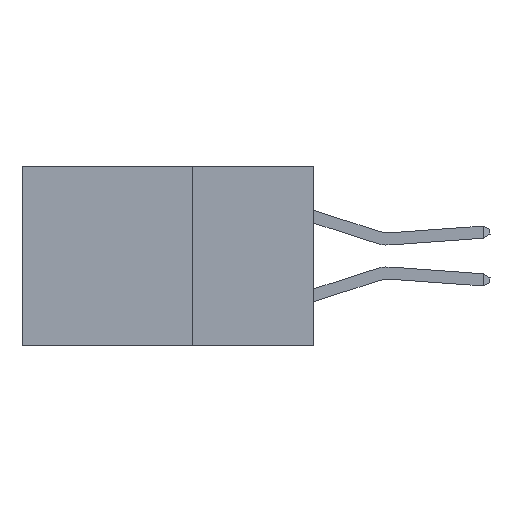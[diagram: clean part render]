
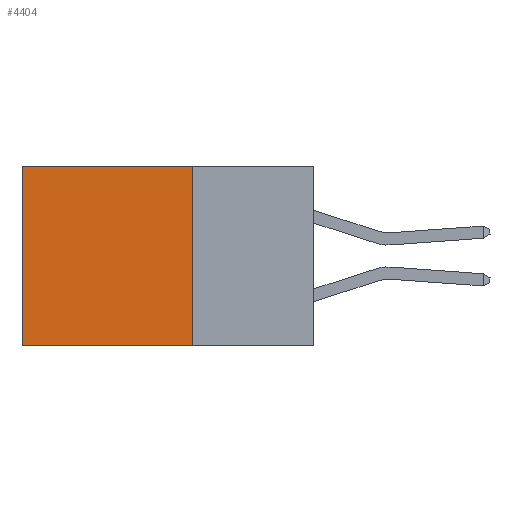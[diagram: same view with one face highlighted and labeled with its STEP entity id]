
A CAD part, left-side view. The second image highlights one B-rep face of the part: STEP entity #4404.
In plain terms, the highlighted planar face has unit normal (-1, 0, 0).
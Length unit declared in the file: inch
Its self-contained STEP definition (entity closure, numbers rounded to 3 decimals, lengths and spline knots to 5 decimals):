
#612 = CARTESIAN_POINT ( 'NONE',  ( 0.2875, 0.6, 0. ) ) ;
#692 = DIRECTION ( 'NONE',  ( 0., 0., -1. ) ) ;
#1323 = DIRECTION ( 'NONE',  ( 0., 1., 0. ) ) ;
#1895 = VERTEX_POINT ( 'NONE', #20215 ) ;
#2215 = ORIENTED_EDGE ( 'NONE', *, *, #22976, .F. ) ;
#2837 = EDGE_CURVE ( 'NONE', #15732, #1895, #19802, .T. ) ;
#3830 = PLANE ( 'NONE',  #8349 ) ;
#3947 = DIRECTION ( 'NONE',  ( 0., 0., -1. ) ) ;
#4209 = VECTOR ( 'NONE', #12485, 39.37008 ) ;
#4404 = ADVANCED_FACE ( 'NONE', ( #16123 ), #3830, .F. ) ;
#5166 = LINE ( 'NONE', #17719, #5786 ) ;
#5183 = CARTESIAN_POINT ( 'NONE',  ( 0.2875, 0.6, 0. ) ) ;
#5786 = VECTOR ( 'NONE', #3947, 39.37008 ) ;
#5808 = DIRECTION ( 'NONE',  ( 1., 0., 0. ) ) ;
#6645 = ORIENTED_EDGE ( 'NONE', *, *, #23198, .F. ) ;
#6925 = VERTEX_POINT ( 'NONE', #11885 ) ;
#7848 = ORIENTED_EDGE ( 'NONE', *, *, #8524, .T. ) ;
#7991 = VERTEX_POINT ( 'NONE', #8976 ) ;
#8349 = AXIS2_PLACEMENT_3D ( 'NONE', #19472, #5808, #19556 ) ;
#8524 = EDGE_CURVE ( 'NONE', #6925, #15732, #14083, .T. ) ;
#8976 = CARTESIAN_POINT ( 'NONE',  ( 0.2875, 0.25, -0.37 ) ) ;
#10125 = VECTOR ( 'NONE', #1323, 39.37008 ) ;
#11139 = CARTESIAN_POINT ( 'NONE',  ( 0.2875, 0.25, -0.37 ) ) ;
#11885 = CARTESIAN_POINT ( 'NONE',  ( 0.2875, 0.25, 0. ) ) ;
#12056 = ORIENTED_EDGE ( 'NONE', *, *, #2837, .T. ) ;
#12402 = CARTESIAN_POINT ( 'NONE',  ( 0.2875, 0.25, 0. ) ) ;
#12485 = DIRECTION ( 'NONE',  ( 0., 1., 0. ) ) ;
#14019 = VECTOR ( 'NONE', #692, 39.37008 ) ;
#14083 = LINE ( 'NONE', #12402, #4209 ) ;
#15391 = LINE ( 'NONE', #11139, #10125 ) ;
#15732 = VERTEX_POINT ( 'NONE', #5183 ) ;
#16123 = FACE_OUTER_BOUND ( 'NONE', #23229, .T. ) ;
#17719 = CARTESIAN_POINT ( 'NONE',  ( 0.2875, 0.25, 0. ) ) ;
#19472 = CARTESIAN_POINT ( 'NONE',  ( 0.2875, 0.25, 0. ) ) ;
#19556 = DIRECTION ( 'NONE',  ( 0., 0., -1. ) ) ;
#19802 = LINE ( 'NONE', #612, #14019 ) ;
#20215 = CARTESIAN_POINT ( 'NONE',  ( 0.2875, 0.6, -0.37 ) ) ;
#22976 = EDGE_CURVE ( 'NONE', #7991, #1895, #15391, .T. ) ;
#23198 = EDGE_CURVE ( 'NONE', #6925, #7991, #5166, .T. ) ;
#23229 = EDGE_LOOP ( 'NONE', ( #12056, #2215, #6645, #7848 ) ) ;
